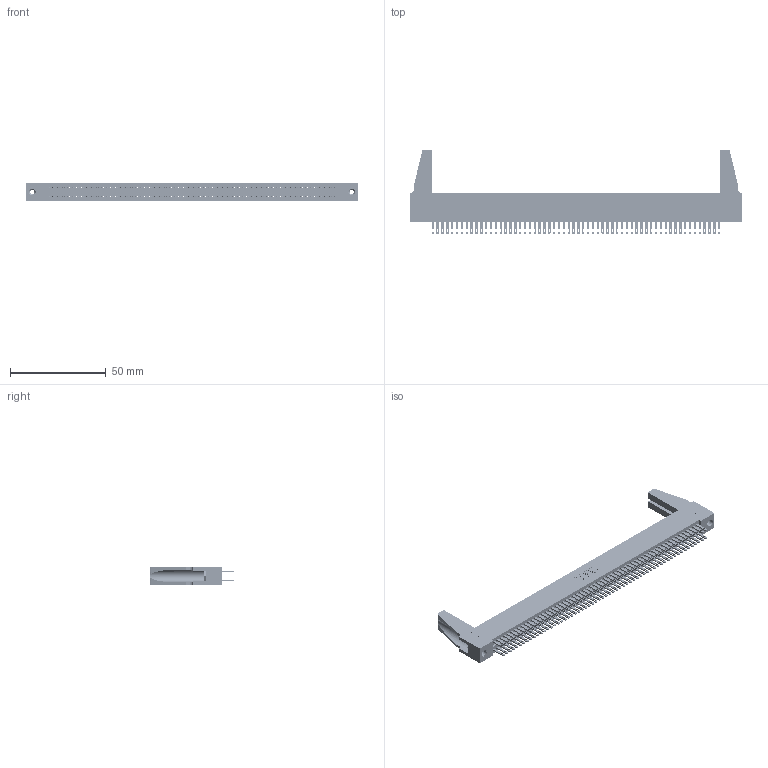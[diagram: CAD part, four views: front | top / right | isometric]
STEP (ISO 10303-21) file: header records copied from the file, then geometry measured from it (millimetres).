
FILE_DESCRIPTION (( 'STEP AP203' ), '1' );
FILE_NAME ('345-120-500-288.STEP', '2019-11-05T23:16:17', ( '' ), ( '' ), 'SwSTEP 2.0', 'SolidWorks 2016', '' );
FILE_SCHEMA (( 'CONFIG_CONTROL_DESIGN' ));
Length unit declared in the file: inch
Products named in the file (5): 345-292-001_345-293-100; 345-250-001_345-250-001-102; 345-120-500-288; 345-220-078_345-220-088; 345 Part_Flush Mounting Lugs - 0.156 Dia-TH
Assembly tree (125 placements, depth 2):
  345-120-500-288
    345 Part_Flush Mounting Lugs - 0.156 Dia-TH
    345-292-001_345-293-100  x120
    345-250-001_345-250-001-102  x2
    345-220-078_345-220-088  x2
Bounding box: 173.63 x 44.37 x 9.4 mm (x, y, z)
Volume: 20653.3 mm3; surface area: 30416 mm2
Topology: 125 solids, 125 shells, 5770 faces, 17575 edges, 11706 vertices
Faces by surface type: plane 3392, cylinder 2362, cone 12, torus 4
Entity records: 46732 total; most frequent: CARTESIAN_POINT 7810, ORIENTED_EDGE 7704, DIRECTION 6872, EDGE_CURVE 3852, LINE 3434, VECTOR 3434, VERTEX_POINT 2562, AXIS2_PLACEMENT_3D 1719
